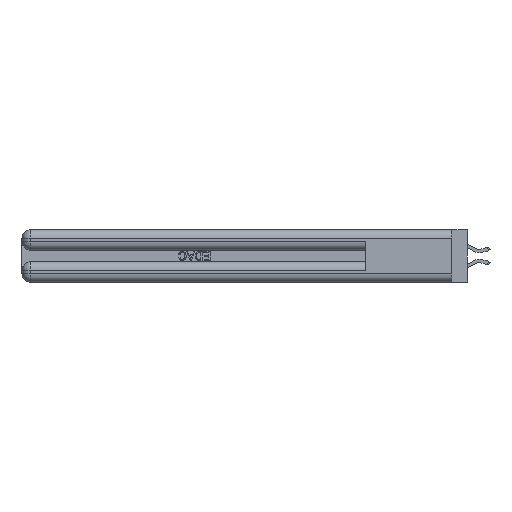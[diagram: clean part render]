
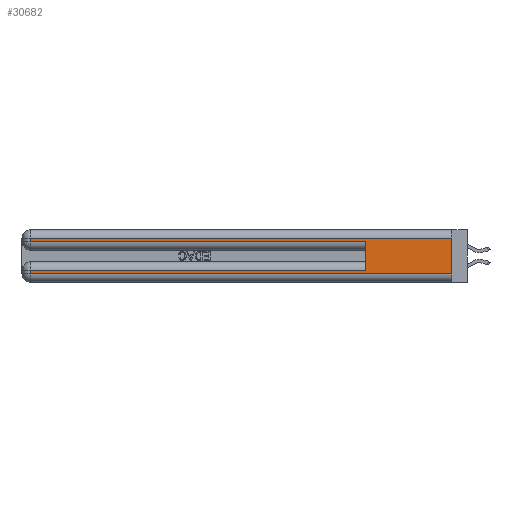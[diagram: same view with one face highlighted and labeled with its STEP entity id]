
A CAD part, left-side view. The second image highlights one B-rep face of the part: STEP entity #30682.
In plain terms, the highlighted planar face has unit normal (-1, 0, 0).
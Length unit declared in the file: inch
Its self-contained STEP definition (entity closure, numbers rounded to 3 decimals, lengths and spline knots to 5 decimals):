
#765 = EDGE_CURVE ( 'NONE', #23721, #2548, #40960, .T. ) ;
#2548 = VERTEX_POINT ( 'NONE', #34409 ) ;
#3298 = ORIENTED_EDGE ( 'NONE', *, *, #26146, .T. ) ;
#3450 = EDGE_CURVE ( 'NONE', #8721, #14689, #16384, .T. ) ;
#3964 = DIRECTION ( 'NONE',  ( 0., 0., -1. ) ) ;
#4147 = VECTOR ( 'NONE', #29085, 39.37008 ) ;
#4540 = ORIENTED_EDGE ( 'NONE', *, *, #765, .F. ) ;
#4636 = DIRECTION ( 'NONE',  ( 0., 0., 1. ) ) ;
#4676 = CARTESIAN_POINT ( 'NONE',  ( 0., 0., 0.06 ) ) ;
#5905 = DIRECTION ( 'NONE',  ( 0., 0., -1. ) ) ;
#6905 = CARTESIAN_POINT ( 'NONE',  ( 0., 0., 0.085 ) ) ;
#7876 = CARTESIAN_POINT ( 'NONE',  ( 0., 2.94, 0.37 ) ) ;
#8606 = VECTOR ( 'NONE', #9126, 39.37008 ) ;
#8721 = VERTEX_POINT ( 'NONE', #30906 ) ;
#9126 = DIRECTION ( 'NONE',  ( 0., 1., 0. ) ) ;
#10220 = VECTOR ( 'NONE', #17146, 39.37008 ) ;
#11247 = DIRECTION ( 'NONE',  ( 0., 0., -1. ) ) ;
#11544 = ORIENTED_EDGE ( 'NONE', *, *, #19877, .T. ) ;
#11603 = VECTOR ( 'NONE', #5905, 39.37008 ) ;
#13403 = VECTOR ( 'NONE', #11247, 39.37008 ) ;
#14689 = VERTEX_POINT ( 'NONE', #4676 ) ;
#15450 = CARTESIAN_POINT ( 'NONE',  ( 0., 2.94, 0.31 ) ) ;
#16241 = CARTESIAN_POINT ( 'NONE',  ( 0., 0., 0.285 ) ) ;
#16384 = LINE ( 'NONE', #24019, #17442 ) ;
#17146 = DIRECTION ( 'NONE',  ( 0., 1., 0. ) ) ;
#17442 = VECTOR ( 'NONE', #3964, 39.37008 ) ;
#17452 = ORIENTED_EDGE ( 'NONE', *, *, #39118, .T. ) ;
#17916 = EDGE_LOOP ( 'NONE', ( #35485, #11544, #17452, #19837, #4540, #19832, #3298, #20816 ) ) ;
#18000 = CARTESIAN_POINT ( 'NONE',  ( 0., 0.6, 0.145 ) ) ;
#18329 = VERTEX_POINT ( 'NONE', #29386 ) ;
#19091 = LINE ( 'NONE', #6905, #10220 ) ;
#19832 = ORIENTED_EDGE ( 'NONE', *, *, #20189, .T. ) ;
#19837 = ORIENTED_EDGE ( 'NONE', *, *, #40310, .T. ) ;
#19877 = EDGE_CURVE ( 'NONE', #8721, #29818, #21123, .T. ) ;
#20189 = EDGE_CURVE ( 'NONE', #23721, #18329, #19091, .T. ) ;
#20334 = VERTEX_POINT ( 'NONE', #25668 ) ;
#20468 = DIRECTION ( 'NONE',  ( 0., 0., -1. ) ) ;
#20816 = ORIENTED_EDGE ( 'NONE', *, *, #39700, .T. ) ;
#21123 = LINE ( 'NONE', #29097, #8606 ) ;
#21762 = AXIS2_PLACEMENT_3D ( 'NONE', #33712, #40305, #20468 ) ;
#22379 = CARTESIAN_POINT ( 'NONE',  ( 0., 0., 0.06 ) ) ;
#23721 = VERTEX_POINT ( 'NONE', #35101 ) ;
#24019 = CARTESIAN_POINT ( 'NONE',  ( 0., 0., 0.37 ) ) ;
#24322 = VERTEX_POINT ( 'NONE', #31757 ) ;
#25668 = CARTESIAN_POINT ( 'NONE',  ( 0., 2.94, 0.285 ) ) ;
#26146 = EDGE_CURVE ( 'NONE', #18329, #24322, #39833, .T. ) ;
#26582 = FACE_OUTER_BOUND ( 'NONE', #17916, .T. ) ;
#27022 = PLANE ( 'NONE',  #21762 ) ;
#29085 = DIRECTION ( 'NONE',  ( 0., -1., 0. ) ) ;
#29097 = CARTESIAN_POINT ( 'NONE',  ( 0., 0., 0.31 ) ) ;
#29283 = CARTESIAN_POINT ( 'NONE',  ( 0., 2.94, 0.37 ) ) ;
#29386 = CARTESIAN_POINT ( 'NONE',  ( 0., 2.94, 0.085 ) ) ;
#29818 = VERTEX_POINT ( 'NONE', #15450 ) ;
#30682 = ADVANCED_FACE ( 'NONE', ( #26582 ), #27022, .F. ) ;
#30816 = LINE ( 'NONE', #22379, #4147 ) ;
#30906 = CARTESIAN_POINT ( 'NONE',  ( 0., 0., 0.31 ) ) ;
#31757 = CARTESIAN_POINT ( 'NONE',  ( 0., 2.94, 0.06 ) ) ;
#32231 = VECTOR ( 'NONE', #4636, 39.37008 ) ;
#33712 = CARTESIAN_POINT ( 'NONE',  ( 0., 0., 0.37 ) ) ;
#34378 = LINE ( 'NONE', #16241, #42070 ) ;
#34409 = CARTESIAN_POINT ( 'NONE',  ( 0., 0.6, 0.285 ) ) ;
#35101 = CARTESIAN_POINT ( 'NONE',  ( 0., 0.6, 0.085 ) ) ;
#35485 = ORIENTED_EDGE ( 'NONE', *, *, #3450, .F. ) ;
#38102 = LINE ( 'NONE', #29283, #11603 ) ;
#39118 = EDGE_CURVE ( 'NONE', #29818, #20334, #38102, .T. ) ;
#39700 = EDGE_CURVE ( 'NONE', #24322, #14689, #30816, .T. ) ;
#39833 = LINE ( 'NONE', #7876, #13403 ) ;
#40305 = DIRECTION ( 'NONE',  ( 1., 0., 0. ) ) ;
#40310 = EDGE_CURVE ( 'NONE', #20334, #2548, #34378, .T. ) ;
#40960 = LINE ( 'NONE', #18000, #32231 ) ;
#42070 = VECTOR ( 'NONE', #42713, 39.37008 ) ;
#42713 = DIRECTION ( 'NONE',  ( 0., -1., 0. ) ) ;
